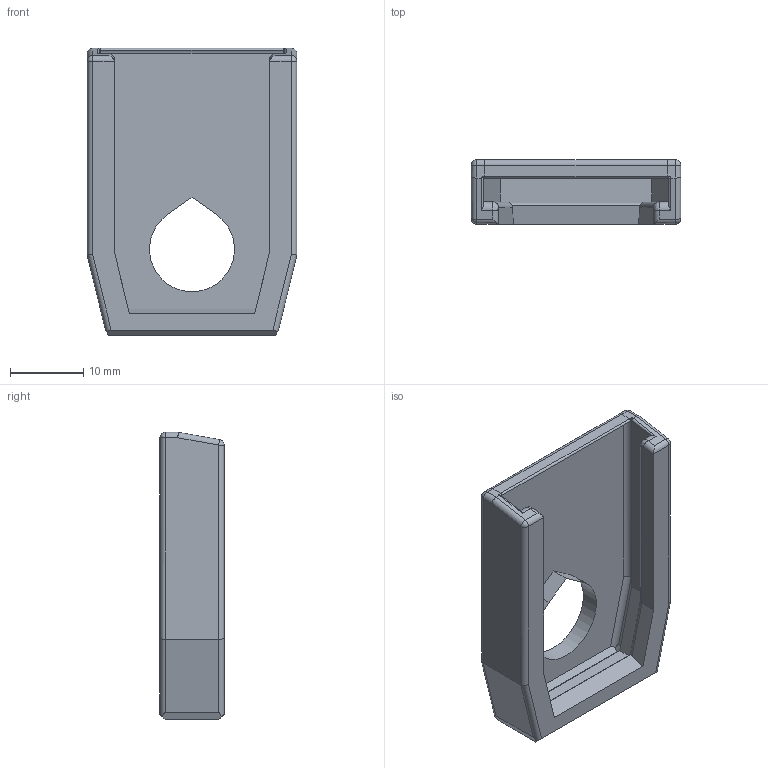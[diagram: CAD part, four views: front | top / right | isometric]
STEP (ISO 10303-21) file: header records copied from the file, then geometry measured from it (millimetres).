
FILE_DESCRIPTION(/* description */ (''),/* implementation_level */ '2;1');
FILE_NAME(/* name */ 'T-Mag M&P Baseplate v1.step',/* time_stamp */ '2022-06-30T09:14:05-05:00',/* author */ (''),/* organization */ (''),/* preprocessor_version */ 'ST-DEVELOPER v19',/* originating_system */ 'Autodesk Translation Framework v11.7.0.108',/* authorisation */ '');
FILE_SCHEMA (('AUTOMOTIVE_DESIGN { 1 0 10303 214 3 1 1 }'));
Length unit declared in the file: millimetre
Products named in the file (1): T-Mag Extended Baseplate
Bounding box: 28.6 x 8.75 x 39.22 mm (x, y, z)
Volume: 3962.5 mm3; surface area: 3860.9 mm2
Topology: 1 solids, 1 shells, 69 faces, 172 edges, 104 vertices
Faces by surface type: cylinder 32, plane 30, sphere 4, bspline 3
Entity records: 2111 total; most frequent: CARTESIAN_POINT 414, DIRECTION 360, ORIENTED_EDGE 342, EDGE_CURVE 171, AXIS2_PLACEMENT_3D 125, LINE 110, VECTOR 110, VERTEX_POINT 104
